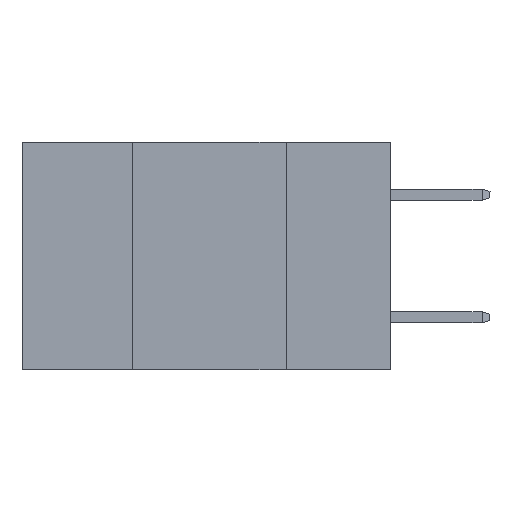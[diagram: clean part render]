
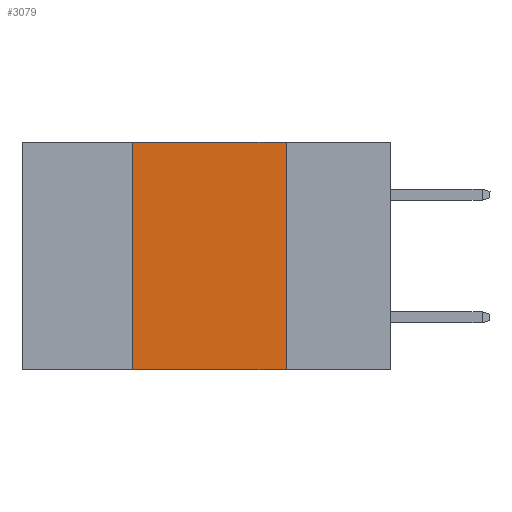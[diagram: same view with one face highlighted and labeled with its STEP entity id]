
A CAD part, left-side view. The second image highlights one B-rep face of the part: STEP entity #3079.
In plain terms, the highlighted planar face has unit normal (-1, 0, 0).
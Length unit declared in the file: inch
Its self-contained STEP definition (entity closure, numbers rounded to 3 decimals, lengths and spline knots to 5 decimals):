
#175 = EDGE_LOOP ( 'NONE', ( #8263, #5921, #5640, #8647 ) ) ;
#253 = CARTESIAN_POINT ( 'NONE',  ( 0., 0.6, 0. ) ) ;
#637 = AXIS2_PLACEMENT_3D ( 'NONE', #7029, #6230, #3862 ) ;
#1564 = LINE ( 'NONE', #9034, #2077 ) ;
#1877 = CARTESIAN_POINT ( 'NONE',  ( 0., 0.42, 0. ) ) ;
#1955 = VECTOR ( 'NONE', #9249, 39.37008 ) ;
#2077 = VECTOR ( 'NONE', #3502, 39.37008 ) ;
#2214 = VECTOR ( 'NONE', #2301, 39.37008 ) ;
#2301 = DIRECTION ( 'NONE',  ( 0., -1., 0. ) ) ;
#2500 = PLANE ( 'NONE',  #637 ) ;
#2738 = LINE ( 'NONE', #10189, #2214 ) ;
#3079 = ADVANCED_FACE ( 'NONE', ( #5152 ), #2500, .F. ) ;
#3502 = DIRECTION ( 'NONE',  ( 0., 0., -1. ) ) ;
#3730 = CARTESIAN_POINT ( 'NONE',  ( 0., 0.42, 0. ) ) ;
#3862 = DIRECTION ( 'NONE',  ( 0., 0., -1. ) ) ;
#3878 = LINE ( 'NONE', #3730, #1955 ) ;
#5093 = VERTEX_POINT ( 'NONE', #5374 ) ;
#5152 = FACE_OUTER_BOUND ( 'NONE', #175, .T. ) ;
#5374 = CARTESIAN_POINT ( 'NONE',  ( 0., 0.17, 0. ) ) ;
#5501 = VERTEX_POINT ( 'NONE', #6532 ) ;
#5640 = ORIENTED_EDGE ( 'NONE', *, *, #7752, .F. ) ;
#5921 = ORIENTED_EDGE ( 'NONE', *, *, #6321, .F. ) ;
#6230 = DIRECTION ( 'NONE',  ( 1., 0., 0. ) ) ;
#6321 = EDGE_CURVE ( 'NONE', #9430, #5093, #7883, .T. ) ;
#6532 = CARTESIAN_POINT ( 'NONE',  ( 0., 0.17, -0.37 ) ) ;
#7029 = CARTESIAN_POINT ( 'NONE',  ( 0., 0.6, 0. ) ) ;
#7241 = EDGE_CURVE ( 'NONE', #8804, #5501, #2738, .T. ) ;
#7752 = EDGE_CURVE ( 'NONE', #8804, #9430, #3878, .T. ) ;
#7883 = LINE ( 'NONE', #253, #8139 ) ;
#8137 = CARTESIAN_POINT ( 'NONE',  ( 0., 0.42, -0.37 ) ) ;
#8139 = VECTOR ( 'NONE', #9948, 39.37008 ) ;
#8263 = ORIENTED_EDGE ( 'NONE', *, *, #8266, .F. ) ;
#8266 = EDGE_CURVE ( 'NONE', #5093, #5501, #1564, .T. ) ;
#8647 = ORIENTED_EDGE ( 'NONE', *, *, #7241, .T. ) ;
#8804 = VERTEX_POINT ( 'NONE', #8137 ) ;
#9034 = CARTESIAN_POINT ( 'NONE',  ( 0., 0.17, 0. ) ) ;
#9249 = DIRECTION ( 'NONE',  ( 0., 0., 1. ) ) ;
#9430 = VERTEX_POINT ( 'NONE', #1877 ) ;
#9948 = DIRECTION ( 'NONE',  ( 0., -1., 0. ) ) ;
#10189 = CARTESIAN_POINT ( 'NONE',  ( 0., 0.6, -0.37 ) ) ;
